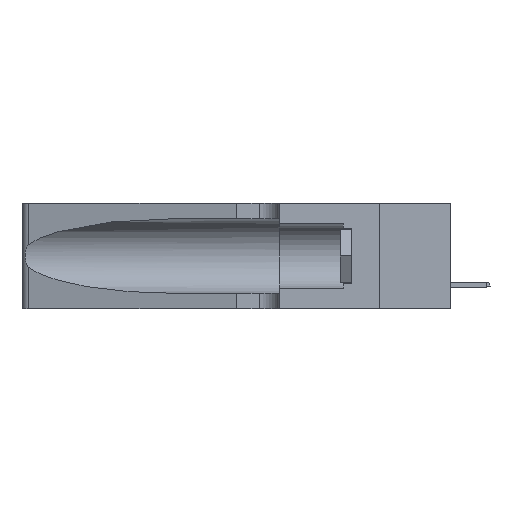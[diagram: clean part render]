
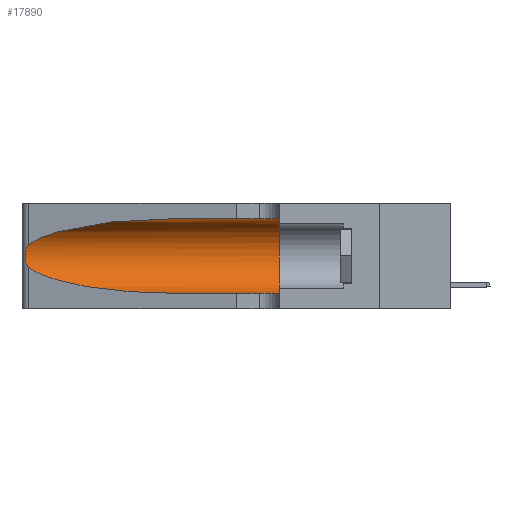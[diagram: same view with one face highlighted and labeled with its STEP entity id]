
A CAD part, left-side view. The second image highlights one B-rep face of the part: STEP entity #17890.
In plain terms, the highlighted cylindrical face has radius 3.308 mm (diameter 6.617 mm), a partial arc.
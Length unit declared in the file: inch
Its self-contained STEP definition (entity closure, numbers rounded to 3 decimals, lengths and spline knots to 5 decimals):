
#285 = VERTEX_POINT ( 'NONE', #11765 ) ;
#1192 = ORIENTED_EDGE ( 'NONE', *, *, #24365, .T. ) ;
#1525 = AXIS2_PLACEMENT_3D ( 'NONE', #24360, #27164, #30608 ) ;
#3558 = VECTOR ( 'NONE', #10093, 39.37008 ) ;
#4683 = DIRECTION ( 'NONE',  ( 0., 0., 1. ) ) ;
#4817 = EDGE_CURVE ( 'NONE', #6835, #20851, #14622, .T. ) ;
#6655 = LINE ( 'NONE', #36531, #3558 ) ;
#6835 = VERTEX_POINT ( 'NONE', #24129 ) ;
#7774 = CARTESIAN_POINT ( 'NONE',  ( 0.25487, 1.22718, 0.14631 ) ) ;
#9776 = CARTESIAN_POINT ( 'NONE',  ( 0.26075, 1.23896, 0.178 ) ) ;
#10093 = DIRECTION ( 'NONE',  ( 0., -1., 0. ) ) ;
#11355 = CARTESIAN_POINT ( 'NONE',  ( 0.1305, 0.35, 0.185 ) ) ;
#11765 = CARTESIAN_POINT ( 'NONE',  ( 0.1305, 0.35, 0.31525 ) ) ;
#12564 = CARTESIAN_POINT ( 'NONE',  ( 0.26017, 1.23833, 0.17102 ) ) ;
#12994 = CARTESIAN_POINT ( 'NONE',  ( 0.25639, 1.23186, 0.15144 ) ) ;
#13213 = CARTESIAN_POINT ( 'NONE',  ( 0.25787, 1.23484, 0.2124 ) ) ;
#13422 = CARTESIAN_POINT ( 'NONE',  ( 0.25555, 1.22994, 0.2215 ) ) ;
#14622 =( BOUNDED_CURVE ( )  B_SPLINE_CURVE ( 3, ( #7774, #40670, #14642, #20891 ),
 .UNSPECIFIED., .F., .T. ) 
 B_SPLINE_CURVE_WITH_KNOTS ( ( 4, 4 ),
 ( 3.44316, 4.71239 ),
 .UNSPECIFIED. ) 
 CURVE ( )  GEOMETRIC_REPRESENTATION_ITEM ( )  RATIONAL_B_SPLINE_CURVE ( ( 1., 0.87, 0.87, 1. ) ) 
 REPRESENTATION_ITEM ( '' )  );
#14642 = CARTESIAN_POINT ( 'NONE',  ( 0.18966, 0.96281, 0.05475 ) ) ;
#14784 = VERTEX_POINT ( 'NONE', #25255 ) ;
#15194 = CARTESIAN_POINT ( 'NONE',  ( 0.2373, 1.15595, 0.28018 ) ) ;
#16219 = CARTESIAN_POINT ( 'NONE',  ( 0.25487, 1.22718, 0.14631 ) ) ;
#16260 = B_SPLINE_CURVE_WITH_KNOTS ( 'NONE', 3,
 ( #29774, #13422, #19878, #13213, #35790, #28912, #42040, #9776, #12564, #22907, #26319, #12994, #36009, #16219 ),
 .UNSPECIFIED., .F., .F.,
 ( 4, 2, 2, 2, 2, 2, 4 ),
 ( 0., 0.00027, 0.00053, 0.00107, 0.0016, 0.00187, 0.00214 ),
 .UNSPECIFIED. ) ;
#17258 = ORIENTED_EDGE ( 'NONE', *, *, #24139, .F. ) ;
#17480 = CYLINDRICAL_SURFACE ( 'NONE', #1525, 0.13025 ) ;
#17786 = EDGE_CURVE ( 'NONE', #38052, #6835, #16260, .T. ) ;
#17890 = ADVANCED_FACE ( 'NONE', ( #30402 ), #17480, .F. ) ;
#18073 = AXIS2_PLACEMENT_3D ( 'NONE', #11355, #24467, #4683 ) ;
#18142 = EDGE_LOOP ( 'NONE', ( #1192, #20248, #24618, #20336, #35639, #17258 ) ) ;
#18658 = CARTESIAN_POINT ( 'NONE',  ( 0.1305, 1.61858, 0.05475 ) ) ;
#19075 = CARTESIAN_POINT ( 'NONE',  ( 0.1305, 0.72297, 0.31525 ) ) ;
#19878 = CARTESIAN_POINT ( 'NONE',  ( 0.25639, 1.23184, 0.21858 ) ) ;
#20248 = ORIENTED_EDGE ( 'NONE', *, *, #17786, .T. ) ;
#20336 = ORIENTED_EDGE ( 'NONE', *, *, #21481, .T. ) ;
#20569 = VECTOR ( 'NONE', #31140, 39.37008 ) ;
#20851 = VERTEX_POINT ( 'NONE', #26479 ) ;
#20891 = CARTESIAN_POINT ( 'NONE',  ( 0.1305, 0.72297, 0.05475 ) ) ;
#21481 = EDGE_CURVE ( 'NONE', #20851, #14784, #27904, .T. ) ;
#22907 = CARTESIAN_POINT ( 'NONE',  ( 0.25856, 1.23593, 0.16098 ) ) ;
#24129 = CARTESIAN_POINT ( 'NONE',  ( 0.25487, 1.22718, 0.14631 ) ) ;
#24139 = EDGE_CURVE ( 'NONE', #34023, #285, #6655, .T. ) ;
#24360 = CARTESIAN_POINT ( 'NONE',  ( 0.1305, 1.61858, 0.185 ) ) ;
#24365 = EDGE_CURVE ( 'NONE', #34023, #38052, #31080, .T. ) ;
#24467 = DIRECTION ( 'NONE',  ( 0., 1., 0. ) ) ;
#24618 = ORIENTED_EDGE ( 'NONE', *, *, #4817, .T. ) ;
#25255 = CARTESIAN_POINT ( 'NONE',  ( 0.1305, 0.35, 0.05475 ) ) ;
#25410 = EDGE_CURVE ( 'NONE', #285, #14784, #29064, .T. ) ;
#25419 = CARTESIAN_POINT ( 'NONE',  ( 0.25487, 1.22718, 0.22369 ) ) ;
#26319 = CARTESIAN_POINT ( 'NONE',  ( 0.25789, 1.23486, 0.15765 ) ) ;
#26479 = CARTESIAN_POINT ( 'NONE',  ( 0.1305, 0.72297, 0.05475 ) ) ;
#27164 = DIRECTION ( 'NONE',  ( 0., -1., 0. ) ) ;
#27904 = LINE ( 'NONE', #18658, #20569 ) ;
#28912 = CARTESIAN_POINT ( 'NONE',  ( 0.26018, 1.23835, 0.19895 ) ) ;
#29064 = CIRCLE ( 'NONE', #18073, 0.13025 ) ;
#29774 = CARTESIAN_POINT ( 'NONE',  ( 0.25487, 1.22718, 0.22369 ) ) ;
#30402 = FACE_OUTER_BOUND ( 'NONE', #18142, .T. ) ;
#30608 = DIRECTION ( 'NONE',  ( 0., 0., -1. ) ) ;
#31080 =( BOUNDED_CURVE ( )  B_SPLINE_CURVE ( 3, ( #19075, #31976, #15194, #34973 ),
 .UNSPECIFIED., .F., .T. ) 
 B_SPLINE_CURVE_WITH_KNOTS ( ( 4, 4 ),
 ( 1.5708, 2.84003 ),
 .UNSPECIFIED. ) 
 CURVE ( )  GEOMETRIC_REPRESENTATION_ITEM ( )  RATIONAL_B_SPLINE_CURVE ( ( 1., 0.87, 0.87, 1. ) ) 
 REPRESENTATION_ITEM ( '' )  );
#31140 = DIRECTION ( 'NONE',  ( 0., -1., 0. ) ) ;
#31976 = CARTESIAN_POINT ( 'NONE',  ( 0.18966, 0.96281, 0.31525 ) ) ;
#34023 = VERTEX_POINT ( 'NONE', #38506 ) ;
#34973 = CARTESIAN_POINT ( 'NONE',  ( 0.25487, 1.22718, 0.22369 ) ) ;
#35639 = ORIENTED_EDGE ( 'NONE', *, *, #25410, .F. ) ;
#35790 = CARTESIAN_POINT ( 'NONE',  ( 0.25854, 1.2359, 0.20912 ) ) ;
#36009 = CARTESIAN_POINT ( 'NONE',  ( 0.25555, 1.22993, 0.14849 ) ) ;
#36531 = CARTESIAN_POINT ( 'NONE',  ( 0.1305, 1.61858, 0.31525 ) ) ;
#38052 = VERTEX_POINT ( 'NONE', #25419 ) ;
#38506 = CARTESIAN_POINT ( 'NONE',  ( 0.1305, 0.72297, 0.31525 ) ) ;
#40670 = CARTESIAN_POINT ( 'NONE',  ( 0.2373, 1.15595, 0.08982 ) ) ;
#42040 = CARTESIAN_POINT ( 'NONE',  ( 0.26075, 1.23896, 0.19203 ) ) ;
